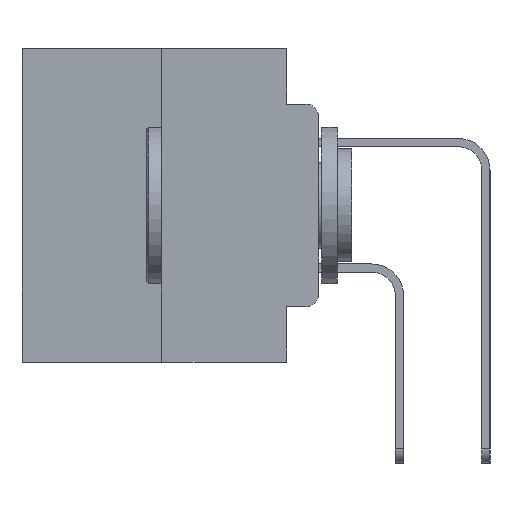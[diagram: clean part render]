
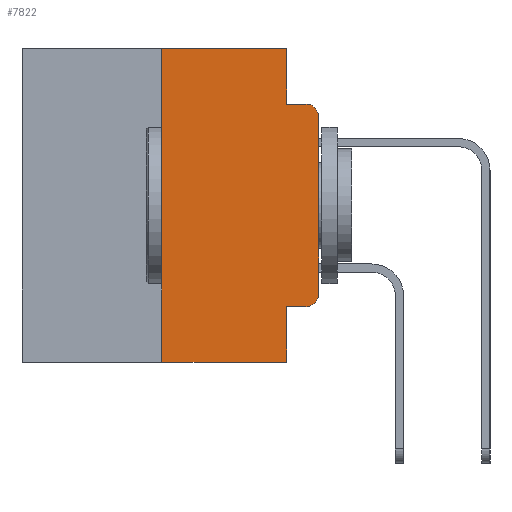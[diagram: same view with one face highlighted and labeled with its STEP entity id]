
A CAD part, left-side view. The second image highlights one B-rep face of the part: STEP entity #7822.
In plain terms, the highlighted planar face has unit normal (-1, 0, 0).
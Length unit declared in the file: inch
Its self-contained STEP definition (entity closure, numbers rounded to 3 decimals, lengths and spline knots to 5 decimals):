
#42 = CARTESIAN_POINT ( 'NONE',  ( 0., 0.25, -0.5 ) ) ;
#503 = VERTEX_POINT ( 'NONE', #27823 ) ;
#873 = CARTESIAN_POINT ( 'NONE',  ( 0., 0.051, 0. ) ) ;
#901 = EDGE_CURVE ( 'NONE', #17434, #11200, #27336, .T. ) ;
#2347 = DIRECTION ( 'NONE',  ( -1., 0., 0. ) ) ;
#2467 = EDGE_CURVE ( 'NONE', #25160, #7522, #11595, .T. ) ;
#3414 = CARTESIAN_POINT ( 'NONE',  ( 0., 0.051, 0. ) ) ;
#3503 = EDGE_LOOP ( 'NONE', ( #3875, #5526, #6672, #7461, #11223, #13438, #14328, #15081, #16280, #16286 ) ) ;
#3875 = ORIENTED_EDGE ( 'NONE', *, *, #23355, .T. ) ;
#3897 = VECTOR ( 'NONE', #11723, 39.37008 ) ;
#3914 = CARTESIAN_POINT ( 'NONE',  ( 0., 0.25, 0. ) ) ;
#4748 = DIRECTION ( 'NONE',  ( 0., 0., 1. ) ) ;
#4924 = DIRECTION ( 'NONE',  ( 0., -1., 0. ) ) ;
#5380 = VERTEX_POINT ( 'NONE', #20096 ) ;
#5406 = CIRCLE ( 'NONE', #22898, 0.02 ) ;
#5526 = ORIENTED_EDGE ( 'NONE', *, *, #14587, .T. ) ;
#5598 = DIRECTION ( 'NONE',  ( 0., 0., -1. ) ) ;
#6064 = CARTESIAN_POINT ( 'NONE',  ( 0., 0.02, -0.1085 ) ) ;
#6653 = VECTOR ( 'NONE', #23373, 39.37008 ) ;
#6672 = ORIENTED_EDGE ( 'NONE', *, *, #13117, .F. ) ;
#7105 = EDGE_CURVE ( 'NONE', #17434, #12197, #16185, .T. ) ;
#7126 = CARTESIAN_POINT ( 'NONE',  ( 0., 0.051, -0.0885 ) ) ;
#7236 = CARTESIAN_POINT ( 'NONE',  ( 0., 0.051, 0. ) ) ;
#7461 = ORIENTED_EDGE ( 'NONE', *, *, #8674, .F. ) ;
#7522 = VERTEX_POINT ( 'NONE', #3914 ) ;
#7822 = ADVANCED_FACE ( 'NONE', ( #25995 ), #24773, .F. ) ;
#8085 = LINE ( 'NONE', #16799, #6653 ) ;
#8349 = DIRECTION ( 'NONE',  ( 0., 0., -1. ) ) ;
#8674 = EDGE_CURVE ( 'NONE', #9114, #27332, #23591, .T. ) ;
#8843 = CARTESIAN_POINT ( 'NONE',  ( 0., 0.051, -0.4115 ) ) ;
#9114 = VERTEX_POINT ( 'NONE', #3414 ) ;
#9830 = VECTOR ( 'NONE', #4748, 39.37008 ) ;
#10589 = VECTOR ( 'NONE', #5598, 39.37008 ) ;
#11200 = VERTEX_POINT ( 'NONE', #26395 ) ;
#11223 = ORIENTED_EDGE ( 'NONE', *, *, #11560, .F. ) ;
#11560 = EDGE_CURVE ( 'NONE', #7522, #9114, #8085, .T. ) ;
#11595 = LINE ( 'NONE', #17217, #16739 ) ;
#11723 = DIRECTION ( 'NONE',  ( 0., 0., -1. ) ) ;
#12197 = VERTEX_POINT ( 'NONE', #17342 ) ;
#13117 = EDGE_CURVE ( 'NONE', #27332, #503, #19351, .T. ) ;
#13438 = ORIENTED_EDGE ( 'NONE', *, *, #2467, .F. ) ;
#13760 = DIRECTION ( 'NONE',  ( 0., -1., 0. ) ) ;
#13922 = DIRECTION ( 'NONE',  ( 0., 0., -1. ) ) ;
#14297 = LINE ( 'NONE', #16888, #9830 ) ;
#14328 = ORIENTED_EDGE ( 'NONE', *, *, #20464, .T. ) ;
#14587 = EDGE_CURVE ( 'NONE', #5380, #503, #27359, .T. ) ;
#14902 = VECTOR ( 'NONE', #4924, 39.37008 ) ;
#15081 = ORIENTED_EDGE ( 'NONE', *, *, #901, .F. ) ;
#15118 = VECTOR ( 'NONE', #25874, 39.37008 ) ;
#15848 = CARTESIAN_POINT ( 'NONE',  ( 0., 0.02, -0.3915 ) ) ;
#16185 = LINE ( 'NONE', #22545, #27027 ) ;
#16280 = ORIENTED_EDGE ( 'NONE', *, *, #7105, .T. ) ;
#16286 = ORIENTED_EDGE ( 'NONE', *, *, #19542, .T. ) ;
#16739 = VECTOR ( 'NONE', #19328, 39.37008 ) ;
#16799 = CARTESIAN_POINT ( 'NONE',  ( 0., 0.473, 0. ) ) ;
#16817 = VERTEX_POINT ( 'NONE', #17816 ) ;
#16888 = CARTESIAN_POINT ( 'NONE',  ( 0., 0., 0. ) ) ;
#17154 = CARTESIAN_POINT ( 'NONE',  ( 0., 0.473, -0.5 ) ) ;
#17217 = CARTESIAN_POINT ( 'NONE',  ( 0., 0.25, 0. ) ) ;
#17342 = CARTESIAN_POINT ( 'NONE',  ( 0., 0.02, -0.4115 ) ) ;
#17434 = VERTEX_POINT ( 'NONE', #8843 ) ;
#17816 = CARTESIAN_POINT ( 'NONE',  ( 0., 0., -0.3915 ) ) ;
#18053 = DIRECTION ( 'NONE',  ( 0., 0., -1. ) ) ;
#19328 = DIRECTION ( 'NONE',  ( 0., 0., 1. ) ) ;
#19351 = LINE ( 'NONE', #20450, #14902 ) ;
#19542 = EDGE_CURVE ( 'NONE', #12197, #16817, #5406, .T. ) ;
#20096 = CARTESIAN_POINT ( 'NONE',  ( 0., 0., -0.1085 ) ) ;
#20450 = CARTESIAN_POINT ( 'NONE',  ( 0., 0.051, -0.0885 ) ) ;
#20464 = EDGE_CURVE ( 'NONE', #25160, #11200, #26647, .T. ) ;
#21534 = DIRECTION ( 'NONE',  ( -1., 0., 0. ) ) ;
#21943 = AXIS2_PLACEMENT_3D ( 'NONE', #6064, #21534, #8349 ) ;
#22516 = CARTESIAN_POINT ( 'NONE',  ( 0., 0.473, 0. ) ) ;
#22545 = CARTESIAN_POINT ( 'NONE',  ( 0., 0.051, -0.4115 ) ) ;
#22898 = AXIS2_PLACEMENT_3D ( 'NONE', #15848, #2347, #18053 ) ;
#23224 = AXIS2_PLACEMENT_3D ( 'NONE', #22516, #26922, #13922 ) ;
#23355 = EDGE_CURVE ( 'NONE', #16817, #5380, #14297, .T. ) ;
#23373 = DIRECTION ( 'NONE',  ( 0., -1., 0. ) ) ;
#23591 = LINE ( 'NONE', #873, #10589 ) ;
#24773 = PLANE ( 'NONE',  #23224 ) ;
#25160 = VERTEX_POINT ( 'NONE', #42 ) ;
#25874 = DIRECTION ( 'NONE',  ( 0., -1., 0. ) ) ;
#25995 = FACE_OUTER_BOUND ( 'NONE', #3503, .T. ) ;
#26395 = CARTESIAN_POINT ( 'NONE',  ( 0., 0.051, -0.5 ) ) ;
#26647 = LINE ( 'NONE', #17154, #15118 ) ;
#26922 = DIRECTION ( 'NONE',  ( 1., 0., 0. ) ) ;
#27027 = VECTOR ( 'NONE', #13760, 39.37008 ) ;
#27332 = VERTEX_POINT ( 'NONE', #7126 ) ;
#27336 = LINE ( 'NONE', #7236, #3897 ) ;
#27359 = CIRCLE ( 'NONE', #21943, 0.02 ) ;
#27823 = CARTESIAN_POINT ( 'NONE',  ( 0., 0.02, -0.0885 ) ) ;
